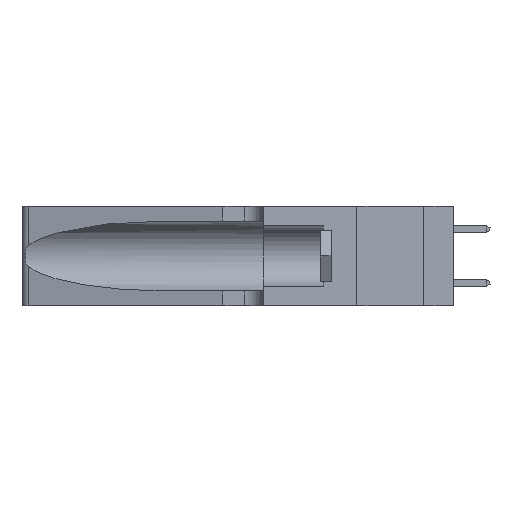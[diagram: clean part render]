
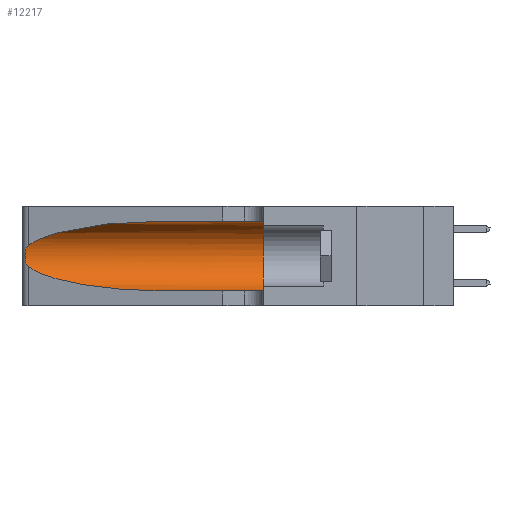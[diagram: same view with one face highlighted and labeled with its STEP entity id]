
A CAD part, left-side view. The second image highlights one B-rep face of the part: STEP entity #12217.
In plain terms, the highlighted cylindrical face has radius 3.308 mm (diameter 6.617 mm), a partial arc.
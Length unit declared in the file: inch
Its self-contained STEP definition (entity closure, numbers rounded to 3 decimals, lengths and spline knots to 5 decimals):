
#331 = CARTESIAN_POINT ( 'NONE',  ( 0.1305, 0.72297, 0.31525 ) ) ;
#729 = CARTESIAN_POINT ( 'NONE',  ( 0.2373, 1.15595, 0.08982 ) ) ;
#905 = VECTOR ( 'NONE', #22515, 39.37008 ) ;
#915 = CARTESIAN_POINT ( 'NONE',  ( 0.26075, 1.23896, 0.19203 ) ) ;
#1990 = DIRECTION ( 'NONE',  ( 0., 1., 0. ) ) ;
#3590 = CYLINDRICAL_SURFACE ( 'NONE', #24408, 0.13025 ) ;
#3967 = CARTESIAN_POINT ( 'NONE',  ( 0.26017, 1.23833, 0.17102 ) ) ;
#4209 = CARTESIAN_POINT ( 'NONE',  ( 0.1305, 1.61858, 0.31525 ) ) ;
#4217 = DIRECTION ( 'NONE',  ( 0., -1., 0. ) ) ;
#5988 = CARTESIAN_POINT ( 'NONE',  ( 0.1305, 0.72297, 0.05475 ) ) ;
#6935 = CARTESIAN_POINT ( 'NONE',  ( 0.25487, 1.22718, 0.22369 ) ) ;
#7075 = CARTESIAN_POINT ( 'NONE',  ( 0.25789, 1.23486, 0.15765 ) ) ;
#7415 = ORIENTED_EDGE ( 'NONE', *, *, #8213, .T. ) ;
#8048 = CARTESIAN_POINT ( 'NONE',  ( 0.1305, 0.35, 0.05475 ) ) ;
#8213 = EDGE_CURVE ( 'NONE', #10722, #20950, #27397, .T. ) ;
#8656 = ORIENTED_EDGE ( 'NONE', *, *, #36464, .T. ) ;
#9144 = ORIENTED_EDGE ( 'NONE', *, *, #14255, .F. ) ;
#9474 = LINE ( 'NONE', #19462, #16649 ) ;
#9647 = AXIS2_PLACEMENT_3D ( 'NONE', #20309, #1990, #23357 ) ;
#9972 = CARTESIAN_POINT ( 'NONE',  ( 0.1305, 0.72297, 0.05475 ) ) ;
#10152 = CARTESIAN_POINT ( 'NONE',  ( 0.25555, 1.22993, 0.14849 ) ) ;
#10346 = B_SPLINE_CURVE_WITH_KNOTS ( 'NONE', 3,
 ( #6935, #25192, #34196, #16179, #37217, #19228, #915, #22287, #3967, #25320, #7075, #28334, #10152, #31313 ),
 .UNSPECIFIED., .F., .F.,
 ( 4, 2, 2, 2, 2, 2, 4 ),
 ( 0., 0.00027, 0.00053, 0.00107, 0.0016, 0.00187, 0.00214 ),
 .UNSPECIFIED. ) ;
#10722 = VERTEX_POINT ( 'NONE', #331 ) ;
#10743 = CARTESIAN_POINT ( 'NONE',  ( 0.25487, 1.22718, 0.22369 ) ) ;
#11535 = CARTESIAN_POINT ( 'NONE',  ( 0.2373, 1.15595, 0.28018 ) ) ;
#12217 = ADVANCED_FACE ( 'NONE', ( #37706 ), #3590, .F. ) ;
#12241 = CARTESIAN_POINT ( 'NONE',  ( 0.1305, 0.35, 0.31525 ) ) ;
#14255 = EDGE_CURVE ( 'NONE', #39116, #21565, #23048, .T. ) ;
#14327 = CARTESIAN_POINT ( 'NONE',  ( 0.1305, 1.61858, 0.185 ) ) ;
#15585 = VERTEX_POINT ( 'NONE', #5988 ) ;
#15841 = EDGE_CURVE ( 'NONE', #15585, #21565, #9474, .T. ) ;
#16179 = CARTESIAN_POINT ( 'NONE',  ( 0.25787, 1.23484, 0.2124 ) ) ;
#16649 = VECTOR ( 'NONE', #4217, 39.37008 ) ;
#16953 = LINE ( 'NONE', #4209, #905 ) ;
#17379 = DIRECTION ( 'NONE',  ( 0., -1., 0. ) ) ;
#17652 = VERTEX_POINT ( 'NONE', #25030 ) ;
#19228 = CARTESIAN_POINT ( 'NONE',  ( 0.26018, 1.23835, 0.19895 ) ) ;
#19462 = CARTESIAN_POINT ( 'NONE',  ( 0.1305, 1.61858, 0.05475 ) ) ;
#20309 = CARTESIAN_POINT ( 'NONE',  ( 0.1305, 0.35, 0.185 ) ) ;
#20950 = VERTEX_POINT ( 'NONE', #10743 ) ;
#21565 = VERTEX_POINT ( 'NONE', #8048 ) ;
#22287 = CARTESIAN_POINT ( 'NONE',  ( 0.26075, 1.23896, 0.178 ) ) ;
#22515 = DIRECTION ( 'NONE',  ( 0., -1., 0. ) ) ;
#23048 = CIRCLE ( 'NONE', #9647, 0.13025 ) ;
#23357 = DIRECTION ( 'NONE',  ( 0., 0., 1. ) ) ;
#24408 = AXIS2_PLACEMENT_3D ( 'NONE', #14327, #17379, #38383 ) ;
#25030 = CARTESIAN_POINT ( 'NONE',  ( 0.25487, 1.22718, 0.14631 ) ) ;
#25192 = CARTESIAN_POINT ( 'NONE',  ( 0.25555, 1.22994, 0.2215 ) ) ;
#25320 = CARTESIAN_POINT ( 'NONE',  ( 0.25856, 1.23593, 0.16098 ) ) ;
#25326 = ORIENTED_EDGE ( 'NONE', *, *, #32981, .F. ) ;
#27397 =( BOUNDED_CURVE ( )  B_SPLINE_CURVE ( 3, ( #35704, #32679, #11535, #38687 ),
 .UNSPECIFIED., .F., .F. ) 
 B_SPLINE_CURVE_WITH_KNOTS ( ( 4, 4 ),
 ( 1.5708, 2.84003 ),
 .UNSPECIFIED. ) 
 CURVE ( )  GEOMETRIC_REPRESENTATION_ITEM ( )  RATIONAL_B_SPLINE_CURVE ( ( 1., 0.87, 0.87, 1. ) ) 
 REPRESENTATION_ITEM ( '' )  );
#28165 = CARTESIAN_POINT ( 'NONE',  ( 0.18966, 0.96281, 0.05475 ) ) ;
#28334 = CARTESIAN_POINT ( 'NONE',  ( 0.25639, 1.23186, 0.15144 ) ) ;
#28590 =( BOUNDED_CURVE ( )  B_SPLINE_CURVE ( 3, ( #37034, #729, #28165, #9972 ),
 .UNSPECIFIED., .F., .T. ) 
 B_SPLINE_CURVE_WITH_KNOTS ( ( 4, 4 ),
 ( 3.44316, 4.71239 ),
 .UNSPECIFIED. ) 
 CURVE ( )  GEOMETRIC_REPRESENTATION_ITEM ( )  RATIONAL_B_SPLINE_CURVE ( ( 1., 0.87, 0.87, 1. ) ) 
 REPRESENTATION_ITEM ( '' )  );
#28965 = ORIENTED_EDGE ( 'NONE', *, *, #29772, .T. ) ;
#29772 = EDGE_CURVE ( 'NONE', #20950, #17652, #10346, .T. ) ;
#30439 = ORIENTED_EDGE ( 'NONE', *, *, #15841, .T. ) ;
#31313 = CARTESIAN_POINT ( 'NONE',  ( 0.25487, 1.22718, 0.14631 ) ) ;
#31514 = EDGE_LOOP ( 'NONE', ( #7415, #28965, #8656, #30439, #9144, #25326 ) ) ;
#32679 = CARTESIAN_POINT ( 'NONE',  ( 0.18966, 0.96281, 0.31525 ) ) ;
#32981 = EDGE_CURVE ( 'NONE', #10722, #39116, #16953, .T. ) ;
#34196 = CARTESIAN_POINT ( 'NONE',  ( 0.25639, 1.23184, 0.21858 ) ) ;
#35704 = CARTESIAN_POINT ( 'NONE',  ( 0.1305, 0.72297, 0.31525 ) ) ;
#36464 = EDGE_CURVE ( 'NONE', #17652, #15585, #28590, .T. ) ;
#37034 = CARTESIAN_POINT ( 'NONE',  ( 0.25487, 1.22718, 0.14631 ) ) ;
#37217 = CARTESIAN_POINT ( 'NONE',  ( 0.25854, 1.2359, 0.20912 ) ) ;
#37706 = FACE_OUTER_BOUND ( 'NONE', #31514, .T. ) ;
#38383 = DIRECTION ( 'NONE',  ( 0., 0., -1. ) ) ;
#38687 = CARTESIAN_POINT ( 'NONE',  ( 0.25487, 1.22718, 0.22369 ) ) ;
#39116 = VERTEX_POINT ( 'NONE', #12241 ) ;
